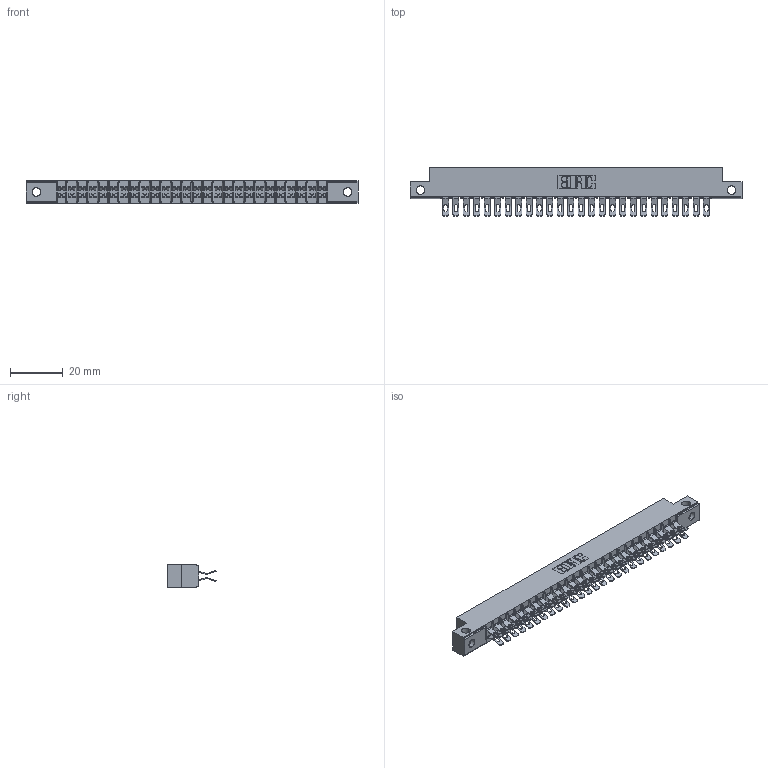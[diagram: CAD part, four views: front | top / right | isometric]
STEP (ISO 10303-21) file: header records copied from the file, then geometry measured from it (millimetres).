
FILE_DESCRIPTION (( 'STEP AP203' ), '1' );
FILE_NAME ('305-052-555-212.STEP', '2020-09-19T22:52:54', ( '' ), ( '' ), 'SwSTEP 2.0', 'SolidWorks 2020', '' );
FILE_SCHEMA (( 'CONFIG_CONTROL_DESIGN' ));
Length unit declared in the file: inch
Products named in the file (3): 305-052-555-212; 305 Part_.128 Dia; 305-290-001_555
Assembly tree (53 placements, depth 2):
  305-052-555-212
    305 Part_.128 Dia
    305-290-001_555  x52
Bounding box: 126.03 x 18.41 x 8.71 mm (x, y, z)
Volume: 7912.5 mm3; surface area: 16065.1 mm2
Topology: 53 solids, 53 shells, 3560 faces, 10622 edges, 6936 vertices
Faces by surface type: plane 1732, cylinder 1724, sphere 104
Entity records: 31129 total; most frequent: CARTESIAN_POINT 5218, ORIENTED_EDGE 5124, DIRECTION 4994, EDGE_CURVE 2562, VECTOR 2018, LINE 2018, VERTEX_POINT 1632, AXIS2_PLACEMENT_3D 1488
